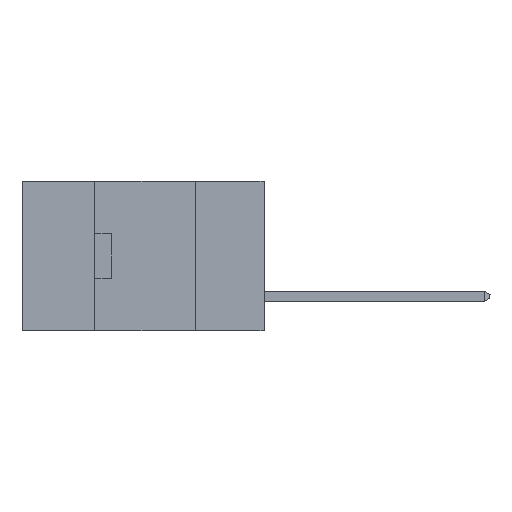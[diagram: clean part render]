
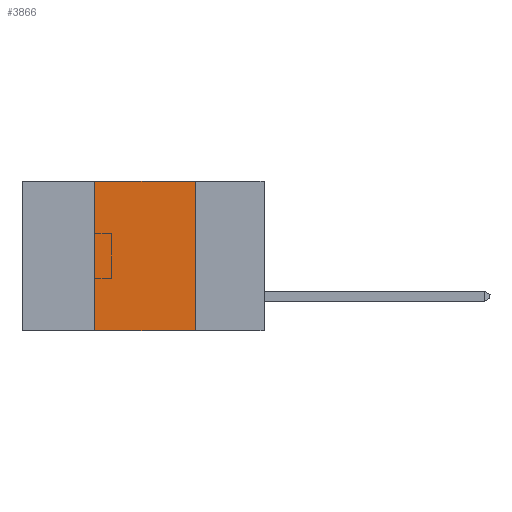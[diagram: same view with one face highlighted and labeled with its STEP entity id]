
A CAD part, left-side view. The second image highlights one B-rep face of the part: STEP entity #3866.
In plain terms, the highlighted planar face has unit normal (-1, 0, 0).
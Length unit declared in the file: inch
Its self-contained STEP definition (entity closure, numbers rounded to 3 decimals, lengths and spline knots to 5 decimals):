
#82 = VECTOR ( 'NONE', #27398, 39.37008 ) ;
#1775 = DIRECTION ( 'NONE',  ( 0., 0., -1. ) ) ;
#3069 = CARTESIAN_POINT ( 'NONE',  ( 0., 0.42, 0. ) ) ;
#3233 = CARTESIAN_POINT ( 'NONE',  ( 0., 0.42, -0.37 ) ) ;
#3523 = VECTOR ( 'NONE', #21910, 39.37008 ) ;
#3854 = LINE ( 'NONE', #12353, #16152 ) ;
#3866 = ADVANCED_FACE ( 'NONE', ( #11571 ), #23818, .F. ) ;
#4730 = CARTESIAN_POINT ( 'NONE',  ( 0., 0.6, 0. ) ) ;
#4782 = LINE ( 'NONE', #24282, #19723 ) ;
#7158 = DIRECTION ( 'NONE',  ( 0., -1., 0. ) ) ;
#8508 = EDGE_LOOP ( 'NONE', ( #23909, #17671, #19623, #14541 ) ) ;
#9631 = VERTEX_POINT ( 'NONE', #3069 ) ;
#10304 = EDGE_CURVE ( 'NONE', #20353, #12830, #3854, .T. ) ;
#11571 = FACE_OUTER_BOUND ( 'NONE', #8508, .T. ) ;
#12029 = EDGE_CURVE ( 'NONE', #26187, #12830, #4782, .T. ) ;
#12353 = CARTESIAN_POINT ( 'NONE',  ( 0., 0.17, -0.37 ) ) ;
#12744 = LINE ( 'NONE', #16805, #82 ) ;
#12830 = VERTEX_POINT ( 'NONE', #18045 ) ;
#13515 = DIRECTION ( 'NONE',  ( 1., 0., 0. ) ) ;
#14541 = ORIENTED_EDGE ( 'NONE', *, *, #12029, .T. ) ;
#15624 = CARTESIAN_POINT ( 'NONE',  ( 0., 0.17, 0. ) ) ;
#15633 = LINE ( 'NONE', #3233, #3523 ) ;
#16152 = VECTOR ( 'NONE', #1775, 39.37008 ) ;
#16211 = AXIS2_PLACEMENT_3D ( 'NONE', #4730, #13515, #17977 ) ;
#16805 = CARTESIAN_POINT ( 'NONE',  ( 0., 0.6, 0. ) ) ;
#17671 = ORIENTED_EDGE ( 'NONE', *, *, #26907, .F. ) ;
#17977 = DIRECTION ( 'NONE',  ( 0., 0., -1. ) ) ;
#18045 = CARTESIAN_POINT ( 'NONE',  ( 0., 0.17, -0.37 ) ) ;
#19623 = ORIENTED_EDGE ( 'NONE', *, *, #24566, .F. ) ;
#19723 = VECTOR ( 'NONE', #7158, 39.37008 ) ;
#20353 = VERTEX_POINT ( 'NONE', #15624 ) ;
#21910 = DIRECTION ( 'NONE',  ( 0., 0., 1. ) ) ;
#23818 = PLANE ( 'NONE',  #16211 ) ;
#23909 = ORIENTED_EDGE ( 'NONE', *, *, #10304, .F. ) ;
#24282 = CARTESIAN_POINT ( 'NONE',  ( 0., 0.6, -0.37 ) ) ;
#24566 = EDGE_CURVE ( 'NONE', #26187, #9631, #15633, .T. ) ;
#26187 = VERTEX_POINT ( 'NONE', #26744 ) ;
#26744 = CARTESIAN_POINT ( 'NONE',  ( 0., 0.42, -0.37 ) ) ;
#26907 = EDGE_CURVE ( 'NONE', #9631, #20353, #12744, .T. ) ;
#27398 = DIRECTION ( 'NONE',  ( 0., -1., 0. ) ) ;
